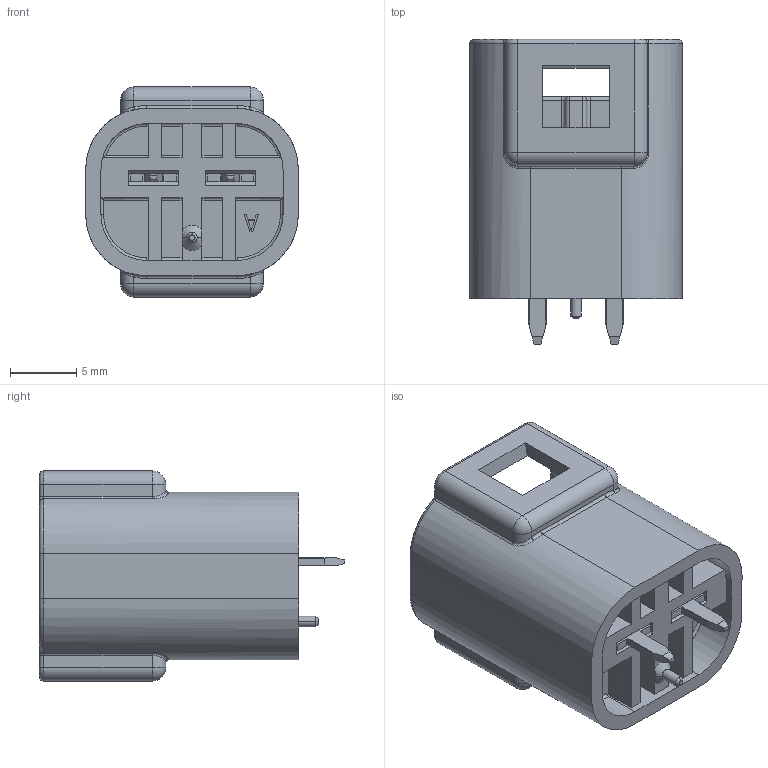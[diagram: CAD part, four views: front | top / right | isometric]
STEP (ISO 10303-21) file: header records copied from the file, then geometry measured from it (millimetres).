
FILE_DESCRIPTION (( 'STEP AP214' ), '1' );
FILE_NAME ('572-002-420-301.STEP', '2020-07-30T18:47:19', ( '' ), ( '' ), 'SwSTEP 2.0', 'SolidWorks 2020', '' );
FILE_SCHEMA (( 'AUTOMOTIVE_DESIGN' ));
Length unit declared in the file: millimetre
Products named in the file (4): 572-002-420-301; 572-002-420-PCB HOUSING_BLUE; 570-420 PCB-TERMINAL-1; 570-420 PCB-TERMINAL-2
Assembly tree (3 placements, depth 2):
  572-002-420-301
    572-002-420-PCB HOUSING_BLUE
    570-420 PCB-TERMINAL-1
    570-420 PCB-TERMINAL-2
Bounding box: 16 x 22.95 x 15.8 mm (x, y, z)
Volume: 1546.5 mm3; surface area: 2757.6 mm2
Topology: 3 solids, 3 shells, 407 faces, 1073 edges, 667 vertices
Faces by surface type: plane 244, cylinder 102, torus 38, sphere 10, cone 9, bspline 4
Entity records: 12732 total; most frequent: CARTESIAN_POINT 2485, ORIENTED_EDGE 2126, DIRECTION 2096, EDGE_CURVE 1063, VECTOR 784, LINE 784, VERTEX_POINT 667, AXIS2_PLACEMENT_3D 656
